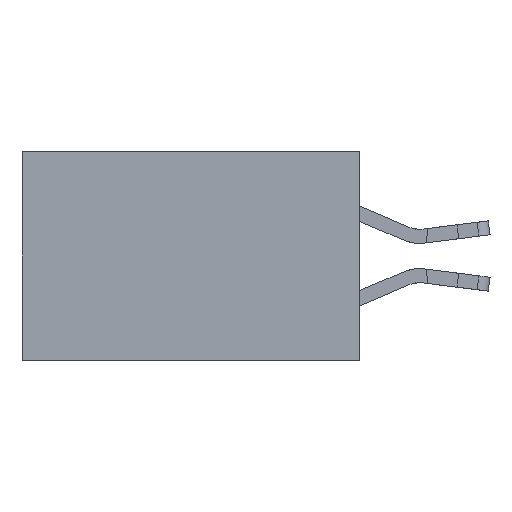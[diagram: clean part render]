
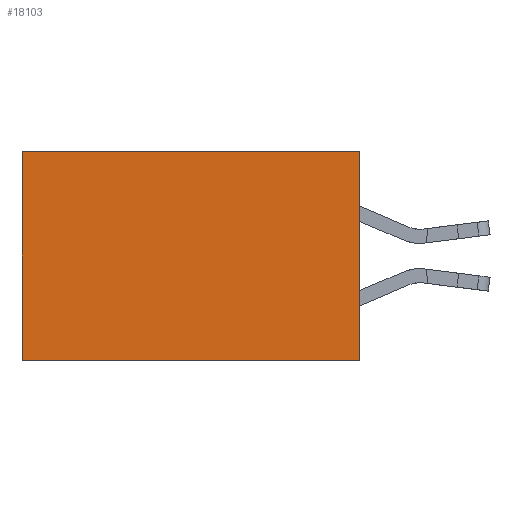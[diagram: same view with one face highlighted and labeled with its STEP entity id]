
A CAD part, left-side view. The second image highlights one B-rep face of the part: STEP entity #18103.
In plain terms, the highlighted planar face has unit normal (-1, 0, 0).
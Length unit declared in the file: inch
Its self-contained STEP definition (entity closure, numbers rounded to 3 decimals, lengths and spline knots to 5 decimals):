
#736 = PLANE ( 'NONE',  #8292 ) ;
#1020 = LINE ( 'NONE', #14053, #12243 ) ;
#1915 = VECTOR ( 'NONE', #14654, 39.37008 ) ;
#4339 = VECTOR ( 'NONE', #24186, 39.37008 ) ;
#5203 = CARTESIAN_POINT ( 'NONE',  ( 0.2875, 0., 0. ) ) ;
#5567 = ORIENTED_EDGE ( 'NONE', *, *, #10675, .T. ) ;
#6445 = CARTESIAN_POINT ( 'NONE',  ( 0.2875, 0., -0.37 ) ) ;
#8292 = AXIS2_PLACEMENT_3D ( 'NONE', #5203, #19186, #19356 ) ;
#8957 = EDGE_LOOP ( 'NONE', ( #12766, #9523, #11920, #5567 ) ) ;
#9208 = VERTEX_POINT ( 'NONE', #23390 ) ;
#9523 = ORIENTED_EDGE ( 'NONE', *, *, #19808, .F. ) ;
#10245 = EDGE_CURVE ( 'NONE', #19241, #10998, #1020, .T. ) ;
#10675 = EDGE_CURVE ( 'NONE', #13541, #19241, #25679, .T. ) ;
#10830 = CARTESIAN_POINT ( 'NONE',  ( 0.2875, 0.6, -0.37 ) ) ;
#10998 = VERTEX_POINT ( 'NONE', #10830 ) ;
#11601 = FACE_OUTER_BOUND ( 'NONE', #8957, .T. ) ;
#11920 = ORIENTED_EDGE ( 'NONE', *, *, #11931, .F. ) ;
#11931 = EDGE_CURVE ( 'NONE', #13541, #9208, #20626, .T. ) ;
#12243 = VECTOR ( 'NONE', #21420, 39.37008 ) ;
#12766 = ORIENTED_EDGE ( 'NONE', *, *, #10245, .T. ) ;
#13541 = VERTEX_POINT ( 'NONE', #23672 ) ;
#14053 = CARTESIAN_POINT ( 'NONE',  ( 0.2875, 0.6, 0. ) ) ;
#14654 = DIRECTION ( 'NONE',  ( 0., 1., 0. ) ) ;
#17676 = CARTESIAN_POINT ( 'NONE',  ( 0.2875, 0., 0. ) ) ;
#18103 = ADVANCED_FACE ( 'NONE', ( #11601 ), #736, .F. ) ;
#19186 = DIRECTION ( 'NONE',  ( 1., 0., 0. ) ) ;
#19241 = VERTEX_POINT ( 'NONE', #20993 ) ;
#19356 = DIRECTION ( 'NONE',  ( 0., 0., -1. ) ) ;
#19808 = EDGE_CURVE ( 'NONE', #9208, #10998, #21773, .T. ) ;
#20626 = LINE ( 'NONE', #22152, #4339 ) ;
#20993 = CARTESIAN_POINT ( 'NONE',  ( 0.2875, 0.6, 0. ) ) ;
#21420 = DIRECTION ( 'NONE',  ( 0., 0., -1. ) ) ;
#21702 = DIRECTION ( 'NONE',  ( 0., 1., 0. ) ) ;
#21773 = LINE ( 'NONE', #6445, #1915 ) ;
#22152 = CARTESIAN_POINT ( 'NONE',  ( 0.2875, 0., 0. ) ) ;
#22753 = VECTOR ( 'NONE', #21702, 39.37008 ) ;
#23390 = CARTESIAN_POINT ( 'NONE',  ( 0.2875, 0., -0.37 ) ) ;
#23672 = CARTESIAN_POINT ( 'NONE',  ( 0.2875, 0., 0. ) ) ;
#24186 = DIRECTION ( 'NONE',  ( 0., 0., -1. ) ) ;
#25679 = LINE ( 'NONE', #17676, #22753 ) ;
